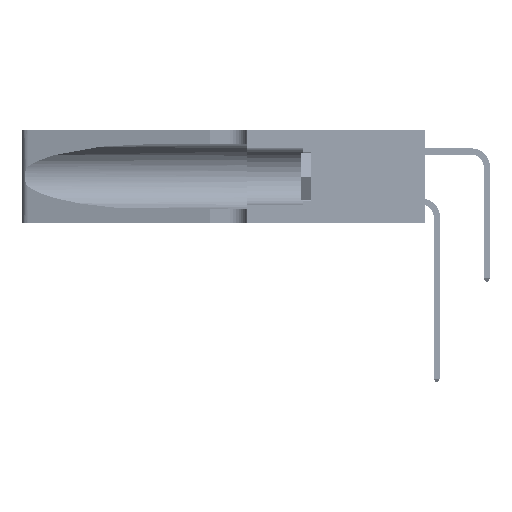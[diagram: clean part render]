
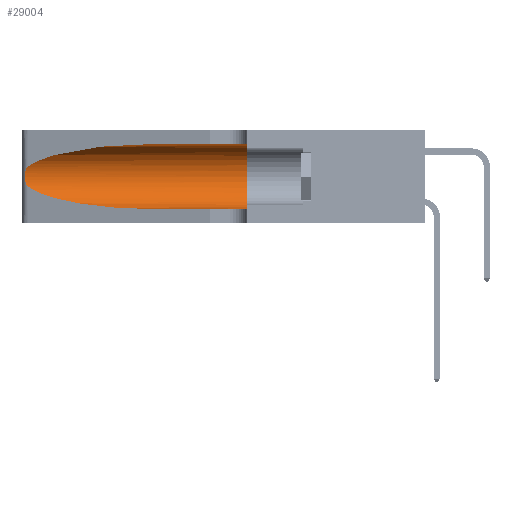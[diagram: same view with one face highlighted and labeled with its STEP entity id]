
A CAD part, left-side view. The second image highlights one B-rep face of the part: STEP entity #29004.
In plain terms, the highlighted cylindrical face has radius 3.308 mm (diameter 6.617 mm), a partial arc.
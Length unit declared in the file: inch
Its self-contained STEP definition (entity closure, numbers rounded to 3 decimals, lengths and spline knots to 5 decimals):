
#306 = ORIENTED_EDGE ( 'NONE', *, *, #18863, .T. ) ;
#1783 = CARTESIAN_POINT ( 'NONE',  ( 0.26017, 1.23833, 0.17102 ) ) ;
#2220 = ORIENTED_EDGE ( 'NONE', *, *, #15804, .F. ) ;
#2473 = CARTESIAN_POINT ( 'NONE',  ( 0.1305, 1.61858, 0.185 ) ) ;
#2912 = VERTEX_POINT ( 'NONE', #12865 ) ;
#3819 = EDGE_LOOP ( 'NONE', ( #11537, #306, #20420, #45631, #42751, #2220 ) ) ;
#5628 = CARTESIAN_POINT ( 'NONE',  ( 0.25789, 1.23486, 0.15765 ) ) ;
#6099 = CARTESIAN_POINT ( 'NONE',  ( 0.25487, 1.22718, 0.14631 ) ) ;
#7080 = VERTEX_POINT ( 'NONE', #45221 ) ;
#8437 = EDGE_CURVE ( 'NONE', #9952, #7080, #23085, .T. ) ;
#8486 = AXIS2_PLACEMENT_3D ( 'NONE', #16052, #42268, #19819 ) ;
#9261 = CARTESIAN_POINT ( 'NONE',  ( 0.25487, 1.22718, 0.22369 ) ) ;
#9386 = LINE ( 'NONE', #14660, #18190 ) ;
#9425 = CARTESIAN_POINT ( 'NONE',  ( 0.25555, 1.22993, 0.14849 ) ) ;
#9526 = CARTESIAN_POINT ( 'NONE',  ( 0.1305, 0.72297, 0.31525 ) ) ;
#9952 = VERTEX_POINT ( 'NONE', #6099 ) ;
#10094 = DIRECTION ( 'NONE',  ( 0., -1., 0. ) ) ;
#11537 = ORIENTED_EDGE ( 'NONE', *, *, #21010, .T. ) ;
#12519 = VERTEX_POINT ( 'NONE', #15708 ) ;
#12865 = CARTESIAN_POINT ( 'NONE',  ( 0.1305, 0.35, 0.05475 ) ) ;
#13019 = CARTESIAN_POINT ( 'NONE',  ( 0.25555, 1.22994, 0.2215 ) ) ;
#14198 = CIRCLE ( 'NONE', #8486, 0.13025 ) ;
#14660 = CARTESIAN_POINT ( 'NONE',  ( 0.1305, 1.61858, 0.05475 ) ) ;
#15322 = CARTESIAN_POINT ( 'NONE',  ( 0.25487, 1.22718, 0.22369 ) ) ;
#15708 = CARTESIAN_POINT ( 'NONE',  ( 0.1305, 0.72297, 0.31525 ) ) ;
#15786 = AXIS2_PLACEMENT_3D ( 'NONE', #2473, #10094, #36326 ) ;
#15804 = EDGE_CURVE ( 'NONE', #12519, #37319, #35618, .T. ) ;
#16052 = CARTESIAN_POINT ( 'NONE',  ( 0.1305, 0.35, 0.185 ) ) ;
#16803 = CARTESIAN_POINT ( 'NONE',  ( 0.25787, 1.23484, 0.2124 ) ) ;
#17077 = CARTESIAN_POINT ( 'NONE',  ( 0.18966, 0.96281, 0.31525 ) ) ;
#18190 = VECTOR ( 'NONE', #40891, 39.37008 ) ;
#18863 = EDGE_CURVE ( 'NONE', #41927, #9952, #28223, .T. ) ;
#18936 = CARTESIAN_POINT ( 'NONE',  ( 0.1305, 0.35, 0.31525 ) ) ;
#19481 =( BOUNDED_CURVE ( )  B_SPLINE_CURVE ( 3, ( #9526, #17077, #20846, #47004 ),
 .UNSPECIFIED., .F., .F. ) 
 B_SPLINE_CURVE_WITH_KNOTS ( ( 4, 4 ),
 ( 1.5708, 2.84003 ),
 .UNSPECIFIED. ) 
 CURVE ( )  GEOMETRIC_REPRESENTATION_ITEM ( )  RATIONAL_B_SPLINE_CURVE ( ( 1., 0.87, 0.87, 1. ) ) 
 REPRESENTATION_ITEM ( '' )  );
#19819 = DIRECTION ( 'NONE',  ( 0., 0., 1. ) ) ;
#19840 = CARTESIAN_POINT ( 'NONE',  ( 0.18966, 0.96281, 0.05475 ) ) ;
#20420 = ORIENTED_EDGE ( 'NONE', *, *, #8437, .T. ) ;
#20567 = CARTESIAN_POINT ( 'NONE',  ( 0.26018, 1.23835, 0.19895 ) ) ;
#20846 = CARTESIAN_POINT ( 'NONE',  ( 0.2373, 1.15595, 0.28018 ) ) ;
#21010 = EDGE_CURVE ( 'NONE', #12519, #41927, #19481, .T. ) ;
#22949 = FACE_OUTER_BOUND ( 'NONE', #3819, .T. ) ;
#23085 =( BOUNDED_CURVE ( )  B_SPLINE_CURVE ( 3, ( #38530, #34757, #19840, #46026 ),
 .UNSPECIFIED., .F., .T. ) 
 B_SPLINE_CURVE_WITH_KNOTS ( ( 4, 4 ),
 ( 3.44316, 4.71239 ),
 .UNSPECIFIED. ) 
 CURVE ( )  GEOMETRIC_REPRESENTATION_ITEM ( )  RATIONAL_B_SPLINE_CURVE ( ( 1., 0.87, 0.87, 1. ) ) 
 REPRESENTATION_ITEM ( '' )  );
#24261 = EDGE_CURVE ( 'NONE', #7080, #2912, #9386, .T. ) ;
#24334 = CARTESIAN_POINT ( 'NONE',  ( 0.26075, 1.23896, 0.178 ) ) ;
#28125 = CARTESIAN_POINT ( 'NONE',  ( 0.25856, 1.23593, 0.16098 ) ) ;
#28223 = B_SPLINE_CURVE_WITH_KNOTS ( 'NONE', 3,
 ( #9261, #13019, #39263, #16803, #43018, #20567, #46746, #24334, #1783, #28125, #5628, #31873, #9425, #35638 ),
 .UNSPECIFIED., .F., .F.,
 ( 4, 2, 2, 2, 2, 2, 4 ),
 ( 0., 0.00027, 0.00053, 0.00107, 0.0016, 0.00187, 0.00214 ),
 .UNSPECIFIED. ) ;
#29004 = ADVANCED_FACE ( 'NONE', ( #22949 ), #41728, .F. ) ;
#31873 = CARTESIAN_POINT ( 'NONE',  ( 0.25639, 1.23186, 0.15144 ) ) ;
#34452 = VECTOR ( 'NONE', #46076, 39.37008 ) ;
#34757 = CARTESIAN_POINT ( 'NONE',  ( 0.2373, 1.15595, 0.08982 ) ) ;
#35618 = LINE ( 'NONE', #42337, #34452 ) ;
#35638 = CARTESIAN_POINT ( 'NONE',  ( 0.25487, 1.22718, 0.14631 ) ) ;
#36326 = DIRECTION ( 'NONE',  ( 0., 0., -1. ) ) ;
#36753 = EDGE_CURVE ( 'NONE', #37319, #2912, #14198, .T. ) ;
#37319 = VERTEX_POINT ( 'NONE', #18936 ) ;
#38530 = CARTESIAN_POINT ( 'NONE',  ( 0.25487, 1.22718, 0.14631 ) ) ;
#39263 = CARTESIAN_POINT ( 'NONE',  ( 0.25639, 1.23184, 0.21858 ) ) ;
#40891 = DIRECTION ( 'NONE',  ( 0., -1., 0. ) ) ;
#41728 = CYLINDRICAL_SURFACE ( 'NONE', #15786, 0.13025 ) ;
#41927 = VERTEX_POINT ( 'NONE', #15322 ) ;
#42268 = DIRECTION ( 'NONE',  ( 0., 1., 0. ) ) ;
#42337 = CARTESIAN_POINT ( 'NONE',  ( 0.1305, 1.61858, 0.31525 ) ) ;
#42751 = ORIENTED_EDGE ( 'NONE', *, *, #36753, .F. ) ;
#43018 = CARTESIAN_POINT ( 'NONE',  ( 0.25854, 1.2359, 0.20912 ) ) ;
#45221 = CARTESIAN_POINT ( 'NONE',  ( 0.1305, 0.72297, 0.05475 ) ) ;
#45631 = ORIENTED_EDGE ( 'NONE', *, *, #24261, .T. ) ;
#46026 = CARTESIAN_POINT ( 'NONE',  ( 0.1305, 0.72297, 0.05475 ) ) ;
#46076 = DIRECTION ( 'NONE',  ( 0., -1., 0. ) ) ;
#46746 = CARTESIAN_POINT ( 'NONE',  ( 0.26075, 1.23896, 0.19203 ) ) ;
#47004 = CARTESIAN_POINT ( 'NONE',  ( 0.25487, 1.22718, 0.22369 ) ) ;
